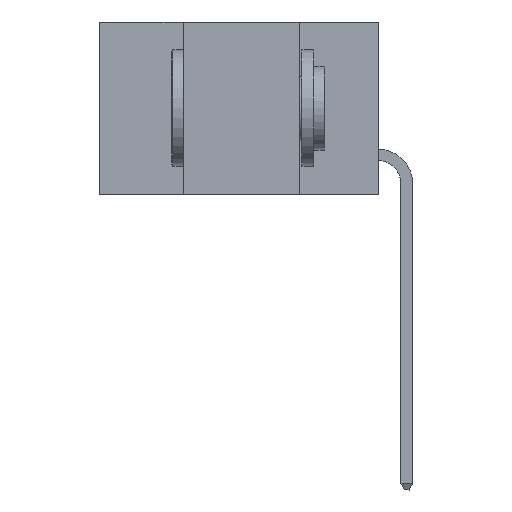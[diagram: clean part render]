
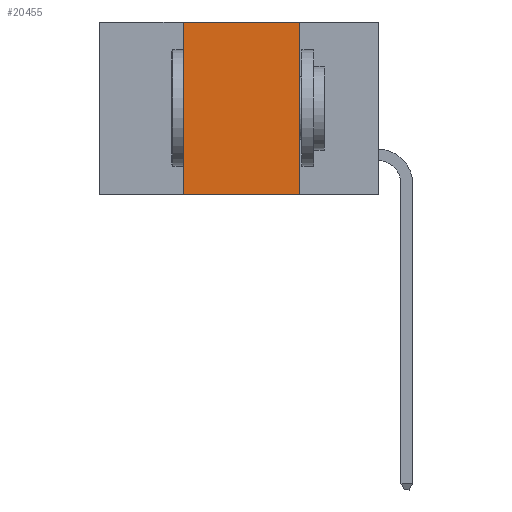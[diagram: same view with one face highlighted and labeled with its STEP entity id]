
A CAD part, left-side view. The second image highlights one B-rep face of the part: STEP entity #20455.
In plain terms, the highlighted planar face has unit normal (-1, 0, 0).
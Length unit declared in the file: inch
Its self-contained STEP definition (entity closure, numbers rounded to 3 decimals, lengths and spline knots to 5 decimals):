
#61 = DIRECTION ( 'NONE',  ( 0., 0., 1. ) ) ;
#591 = VERTEX_POINT ( 'NONE', #9782 ) ;
#1264 = VECTOR ( 'NONE', #8641, 39.37008 ) ;
#2096 = CARTESIAN_POINT ( 'NONE',  ( 0., 0.42, 0. ) ) ;
#2137 = ORIENTED_EDGE ( 'NONE', *, *, #9159, .F. ) ;
#3338 = DIRECTION ( 'NONE',  ( 0., -1., 0. ) ) ;
#5071 = PLANE ( 'NONE',  #23210 ) ;
#5527 = DIRECTION ( 'NONE',  ( 0., -1., 0. ) ) ;
#6032 = LINE ( 'NONE', #24033, #17290 ) ;
#6566 = VERTEX_POINT ( 'NONE', #2096 ) ;
#7229 = ORIENTED_EDGE ( 'NONE', *, *, #19456, .F. ) ;
#7742 = CARTESIAN_POINT ( 'NONE',  ( 0., 0.17, -0.37 ) ) ;
#8641 = DIRECTION ( 'NONE',  ( 0., 0., -1. ) ) ;
#9031 = EDGE_CURVE ( 'NONE', #6566, #591, #17039, .T. ) ;
#9159 = EDGE_CURVE ( 'NONE', #17654, #6566, #6032, .T. ) ;
#9293 = DIRECTION ( 'NONE',  ( 1., 0., 0. ) ) ;
#9782 = CARTESIAN_POINT ( 'NONE',  ( 0., 0.17, 0. ) ) ;
#10254 = EDGE_LOOP ( 'NONE', ( #7229, #24864, #2137, #11913 ) ) ;
#11913 = ORIENTED_EDGE ( 'NONE', *, *, #13528, .T. ) ;
#12263 = VECTOR ( 'NONE', #3338, 39.37008 ) ;
#13085 = CARTESIAN_POINT ( 'NONE',  ( 0., 0.17, -0.37 ) ) ;
#13528 = EDGE_CURVE ( 'NONE', #17654, #24728, #25215, .T. ) ;
#14074 = CARTESIAN_POINT ( 'NONE',  ( 0., 0.42, -0.37 ) ) ;
#15097 = CARTESIAN_POINT ( 'NONE',  ( 0., 0.6, 0. ) ) ;
#17039 = LINE ( 'NONE', #15097, #18129 ) ;
#17290 = VECTOR ( 'NONE', #61, 39.37008 ) ;
#17357 = FACE_OUTER_BOUND ( 'NONE', #10254, .T. ) ;
#17654 = VERTEX_POINT ( 'NONE', #14074 ) ;
#18129 = VECTOR ( 'NONE', #5527, 39.37008 ) ;
#18926 = CARTESIAN_POINT ( 'NONE',  ( 0., 0.6, 0. ) ) ;
#19456 = EDGE_CURVE ( 'NONE', #591, #24728, #25505, .T. ) ;
#20455 = ADVANCED_FACE ( 'NONE', ( #17357 ), #5071, .F. ) ;
#21084 = CARTESIAN_POINT ( 'NONE',  ( 0., 0.6, -0.37 ) ) ;
#23210 = AXIS2_PLACEMENT_3D ( 'NONE', #18926, #9293, #24770 ) ;
#24033 = CARTESIAN_POINT ( 'NONE',  ( 0., 0.42, -0.37 ) ) ;
#24728 = VERTEX_POINT ( 'NONE', #13085 ) ;
#24770 = DIRECTION ( 'NONE',  ( 0., 0., -1. ) ) ;
#24864 = ORIENTED_EDGE ( 'NONE', *, *, #9031, .F. ) ;
#25215 = LINE ( 'NONE', #21084, #12263 ) ;
#25505 = LINE ( 'NONE', #7742, #1264 ) ;
